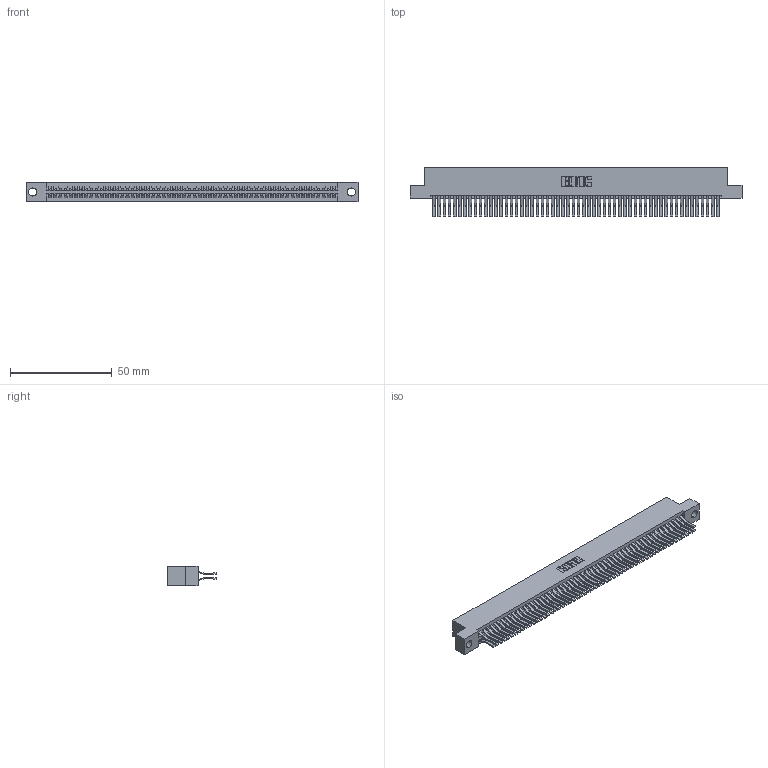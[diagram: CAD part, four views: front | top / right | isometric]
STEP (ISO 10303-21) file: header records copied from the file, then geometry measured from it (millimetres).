
FILE_DESCRIPTION (( 'STEP AP203' ), '1' );
FILE_NAME ('345-112-560-204.STEP', '2018-10-07T17:44:03', ( '' ), ( '' ), 'SwSTEP 2.0', 'SolidWorks 2016', '' );
FILE_SCHEMA (( 'CONFIG_CONTROL_DESIGN' ));
Length unit declared in the file: inch
Products named in the file (3): 345-112-560-204; 345 Part_Flush Mounting Lugs - 0.156 Dia-TH; 345-292-001_560 Tail
Assembly tree (113 placements, depth 2):
  345-112-560-204
    345 Part_Flush Mounting Lugs - 0.156 Dia-TH
    345-292-001_560 Tail  x112
Bounding box: 163.45 x 24.45 x 9.4 mm (x, y, z)
Volume: 16653.8 mm3; surface area: 26591.5 mm2
Topology: 113 solids, 113 shells, 5950 faces, 17701 edges, 11650 vertices
Faces by surface type: plane 3776, cylinder 2174
Entity records: 42145 total; most frequent: CARTESIAN_POINT 7052, ORIENTED_EDGE 6986, DIRECTION 6205, EDGE_CURVE 3493, VECTOR 3133, LINE 3133, VERTEX_POINT 2326, AXIS2_PLACEMENT_3D 1536
